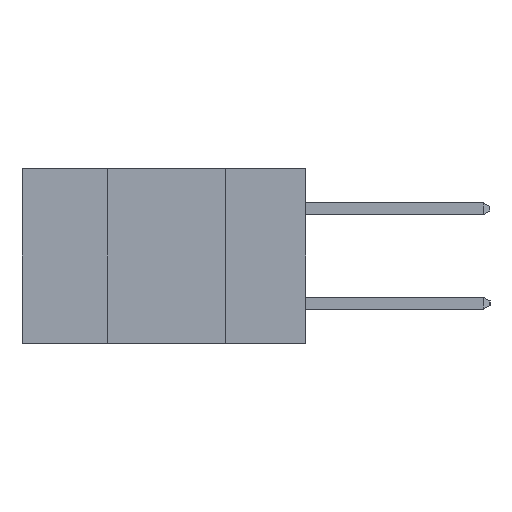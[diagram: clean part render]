
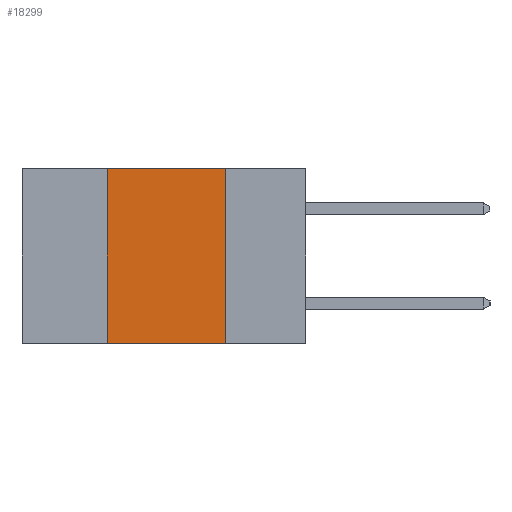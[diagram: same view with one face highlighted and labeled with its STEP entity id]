
A CAD part, left-side view. The second image highlights one B-rep face of the part: STEP entity #18299.
In plain terms, the highlighted planar face has unit normal (-1, 0, 0).
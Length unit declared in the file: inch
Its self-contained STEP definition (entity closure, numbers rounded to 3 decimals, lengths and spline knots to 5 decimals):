
#1163 = DIRECTION ( 'NONE',  ( 0., -1., 0. ) ) ;
#1314 = DIRECTION ( 'NONE',  ( 0., 0., -1. ) ) ;
#1409 = EDGE_CURVE ( 'NONE', #17915, #13537, #7210, .T. ) ;
#1607 = LINE ( 'NONE', #8545, #20125 ) ;
#2741 = PLANE ( 'NONE',  #19112 ) ;
#2794 = CARTESIAN_POINT ( 'NONE',  ( 0., 0.17, 0. ) ) ;
#3527 = CARTESIAN_POINT ( 'NONE',  ( 0., 0.6, -0.37 ) ) ;
#3854 = EDGE_CURVE ( 'NONE', #17915, #3887, #15201, .T. ) ;
#3887 = VERTEX_POINT ( 'NONE', #20410 ) ;
#6064 = ORIENTED_EDGE ( 'NONE', *, *, #18711, .F. ) ;
#6659 = VECTOR ( 'NONE', #1163, 39.37008 ) ;
#7210 = LINE ( 'NONE', #3527, #6659 ) ;
#7837 = DIRECTION ( 'NONE',  ( 0., 0., 1. ) ) ;
#7887 = VERTEX_POINT ( 'NONE', #2794 ) ;
#8118 = DIRECTION ( 'NONE',  ( 1., 0., 0. ) ) ;
#8196 = CARTESIAN_POINT ( 'NONE',  ( 0., 0.17, -0.37 ) ) ;
#8545 = CARTESIAN_POINT ( 'NONE',  ( 0., 0.6, 0. ) ) ;
#8593 = CARTESIAN_POINT ( 'NONE',  ( 0., 0.42, -0.37 ) ) ;
#9687 = ORIENTED_EDGE ( 'NONE', *, *, #22260, .F. ) ;
#9877 = VECTOR ( 'NONE', #1314, 39.37008 ) ;
#11345 = ORIENTED_EDGE ( 'NONE', *, *, #3854, .F. ) ;
#11916 = ORIENTED_EDGE ( 'NONE', *, *, #1409, .T. ) ;
#13129 = CARTESIAN_POINT ( 'NONE',  ( 0., 0.42, -0.37 ) ) ;
#13537 = VERTEX_POINT ( 'NONE', #8196 ) ;
#13992 = DIRECTION ( 'NONE',  ( 0., -1., 0. ) ) ;
#14620 = VECTOR ( 'NONE', #7837, 39.37008 ) ;
#15201 = LINE ( 'NONE', #13129, #14620 ) ;
#16790 = FACE_OUTER_BOUND ( 'NONE', #22008, .T. ) ;
#17915 = VERTEX_POINT ( 'NONE', #8593 ) ;
#18299 = ADVANCED_FACE ( 'NONE', ( #16790 ), #2741, .F. ) ;
#18711 = EDGE_CURVE ( 'NONE', #3887, #7887, #1607, .T. ) ;
#18850 = CARTESIAN_POINT ( 'NONE',  ( 0., 0.6, 0. ) ) ;
#19112 = AXIS2_PLACEMENT_3D ( 'NONE', #18850, #8118, #20624 ) ;
#19400 = LINE ( 'NONE', #22766, #9877 ) ;
#20125 = VECTOR ( 'NONE', #13992, 39.37008 ) ;
#20410 = CARTESIAN_POINT ( 'NONE',  ( 0., 0.42, 0. ) ) ;
#20624 = DIRECTION ( 'NONE',  ( 0., 0., -1. ) ) ;
#22008 = EDGE_LOOP ( 'NONE', ( #9687, #6064, #11345, #11916 ) ) ;
#22260 = EDGE_CURVE ( 'NONE', #7887, #13537, #19400, .T. ) ;
#22766 = CARTESIAN_POINT ( 'NONE',  ( 0., 0.17, -0.37 ) ) ;
